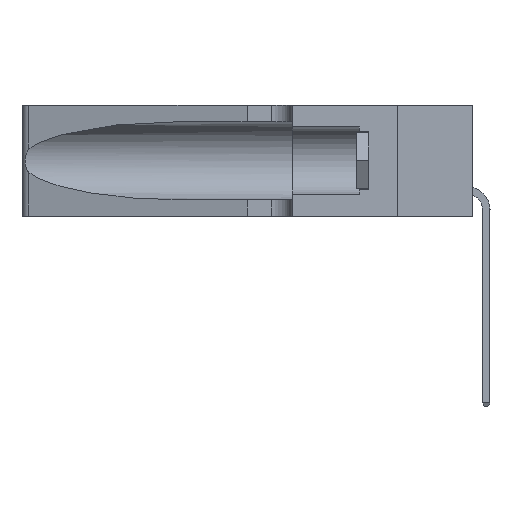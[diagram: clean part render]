
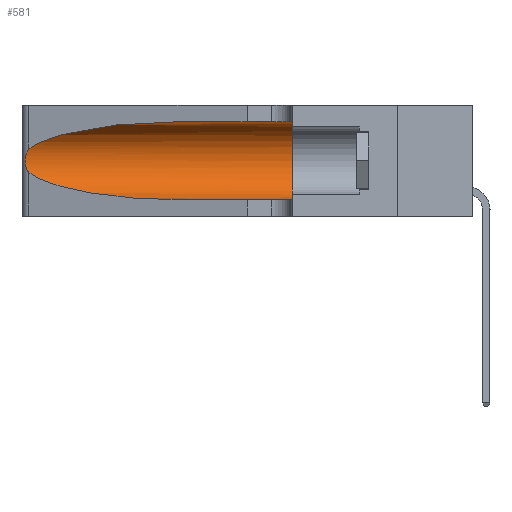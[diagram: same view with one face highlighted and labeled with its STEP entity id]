
A CAD part, left-side view. The second image highlights one B-rep face of the part: STEP entity #581.
In plain terms, the highlighted cylindrical face has radius 3.308 mm (diameter 6.617 mm), a partial arc.
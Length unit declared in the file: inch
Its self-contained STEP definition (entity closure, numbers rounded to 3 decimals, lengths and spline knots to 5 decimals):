
#228 = EDGE_CURVE ( 'NONE', #7086, #34649, #12203, .T. ) ;
#581 = ADVANCED_FACE ( 'NONE', ( #31337 ), #18608, .F. ) ;
#1753 = CARTESIAN_POINT ( 'NONE',  ( 0.25639, 1.23186, 0.15144 ) ) ;
#2280 =( BOUNDED_CURVE ( )  B_SPLINE_CURVE ( 3, ( #18532, #28367, #24804, #37638 ),
 .UNSPECIFIED., .F., .T. ) 
 B_SPLINE_CURVE_WITH_KNOTS ( ( 4, 4 ),
 ( 1.5708, 2.84003 ),
 .UNSPECIFIED. ) 
 CURVE ( )  GEOMETRIC_REPRESENTATION_ITEM ( )  RATIONAL_B_SPLINE_CURVE ( ( 1., 0.87, 0.87, 1. ) ) 
 REPRESENTATION_ITEM ( '' )  );
#4616 =( BOUNDED_CURVE ( )  B_SPLINE_CURVE ( 3, ( #35679, #6093, #32330, #28682 ),
 .UNSPECIFIED., .F., .F. ) 
 B_SPLINE_CURVE_WITH_KNOTS ( ( 4, 4 ),
 ( 3.44316, 4.71239 ),
 .UNSPECIFIED. ) 
 CURVE ( )  GEOMETRIC_REPRESENTATION_ITEM ( )  RATIONAL_B_SPLINE_CURVE ( ( 1., 0.87, 0.87, 1. ) ) 
 REPRESENTATION_ITEM ( '' )  );
#4776 = EDGE_CURVE ( 'NONE', #40085, #14666, #27175, .T. ) ;
#5029 = CARTESIAN_POINT ( 'NONE',  ( 0.25789, 1.23486, 0.15765 ) ) ;
#6093 = CARTESIAN_POINT ( 'NONE',  ( 0.2373, 1.15595, 0.08982 ) ) ;
#7025 = CARTESIAN_POINT ( 'NONE',  ( 0.25555, 1.22994, 0.2215 ) ) ;
#7086 = VERTEX_POINT ( 'NONE', #40949 ) ;
#7483 = ORIENTED_EDGE ( 'NONE', *, *, #8752, .T. ) ;
#8303 = CARTESIAN_POINT ( 'NONE',  ( 0.25555, 1.22993, 0.14849 ) ) ;
#8752 = EDGE_CURVE ( 'NONE', #40085, #7086, #2280, .T. ) ;
#9869 = CARTESIAN_POINT ( 'NONE',  ( 0.1305, 1.61858, 0.31525 ) ) ;
#10155 = ORIENTED_EDGE ( 'NONE', *, *, #11178, .T. ) ;
#11040 = VECTOR ( 'NONE', #30223, 39.37008 ) ;
#11178 = EDGE_CURVE ( 'NONE', #22840, #31168, #31362, .T. ) ;
#12203 = B_SPLINE_CURVE_WITH_KNOTS ( 'NONE', 3,
 ( #30043, #7025, #39729, #36611, #32995, #21078, #37460, #14257, #30453, #37320, #5029, #1753, #8303, #31007 ),
 .UNSPECIFIED., .F., .F.,
 ( 4, 2, 2, 2, 2, 2, 4 ),
 ( 0., 0.00027, 0.00053, 0.00107, 0.0016, 0.00187, 0.00214 ),
 .UNSPECIFIED. ) ;
#14257 = CARTESIAN_POINT ( 'NONE',  ( 0.26075, 1.23896, 0.178 ) ) ;
#14320 = CIRCLE ( 'NONE', #38857, 0.13025 ) ;
#14666 = VERTEX_POINT ( 'NONE', #34007 ) ;
#17607 = CARTESIAN_POINT ( 'NONE',  ( 0.25487, 1.22718, 0.14631 ) ) ;
#18046 = CARTESIAN_POINT ( 'NONE',  ( 0.1305, 1.61858, 0.185 ) ) ;
#18532 = CARTESIAN_POINT ( 'NONE',  ( 0.1305, 0.72297, 0.31525 ) ) ;
#18549 = VECTOR ( 'NONE', #25779, 39.37008 ) ;
#18608 = CYLINDRICAL_SURFACE ( 'NONE', #26297, 0.13025 ) ;
#18941 = CARTESIAN_POINT ( 'NONE',  ( 0.1305, 0.35, 0.185 ) ) ;
#19508 = DIRECTION ( 'NONE',  ( 0., 0., 1. ) ) ;
#20144 = CARTESIAN_POINT ( 'NONE',  ( 0.1305, 1.61858, 0.05475 ) ) ;
#21078 = CARTESIAN_POINT ( 'NONE',  ( 0.26018, 1.23835, 0.19895 ) ) ;
#22840 = VERTEX_POINT ( 'NONE', #32317 ) ;
#23544 = CARTESIAN_POINT ( 'NONE',  ( 0.1305, 0.35, 0.05475 ) ) ;
#23941 = EDGE_LOOP ( 'NONE', ( #7483, #37481, #27740, #10155, #29440, #30219 ) ) ;
#24804 = CARTESIAN_POINT ( 'NONE',  ( 0.2373, 1.15595, 0.28018 ) ) ;
#25779 = DIRECTION ( 'NONE',  ( 0., -1., 0. ) ) ;
#25839 = EDGE_CURVE ( 'NONE', #14666, #31168, #14320, .T. ) ;
#26297 = AXIS2_PLACEMENT_3D ( 'NONE', #18046, #27987, #31938 ) ;
#27175 = LINE ( 'NONE', #9869, #18549 ) ;
#27740 = ORIENTED_EDGE ( 'NONE', *, *, #39529, .T. ) ;
#27987 = DIRECTION ( 'NONE',  ( 0., -1., 0. ) ) ;
#28367 = CARTESIAN_POINT ( 'NONE',  ( 0.18966, 0.96281, 0.31525 ) ) ;
#28682 = CARTESIAN_POINT ( 'NONE',  ( 0.1305, 0.72297, 0.05475 ) ) ;
#29440 = ORIENTED_EDGE ( 'NONE', *, *, #25839, .F. ) ;
#30043 = CARTESIAN_POINT ( 'NONE',  ( 0.25487, 1.22718, 0.22369 ) ) ;
#30219 = ORIENTED_EDGE ( 'NONE', *, *, #4776, .F. ) ;
#30223 = DIRECTION ( 'NONE',  ( 0., -1., 0. ) ) ;
#30453 = CARTESIAN_POINT ( 'NONE',  ( 0.26017, 1.23833, 0.17102 ) ) ;
#31007 = CARTESIAN_POINT ( 'NONE',  ( 0.25487, 1.22718, 0.14631 ) ) ;
#31168 = VERTEX_POINT ( 'NONE', #23544 ) ;
#31337 = FACE_OUTER_BOUND ( 'NONE', #23941, .T. ) ;
#31362 = LINE ( 'NONE', #20144, #11040 ) ;
#31588 = CARTESIAN_POINT ( 'NONE',  ( 0.1305, 0.72297, 0.31525 ) ) ;
#31938 = DIRECTION ( 'NONE',  ( 0., 0., -1. ) ) ;
#32144 = DIRECTION ( 'NONE',  ( 0., 1., 0. ) ) ;
#32317 = CARTESIAN_POINT ( 'NONE',  ( 0.1305, 0.72297, 0.05475 ) ) ;
#32330 = CARTESIAN_POINT ( 'NONE',  ( 0.18966, 0.96281, 0.05475 ) ) ;
#32995 = CARTESIAN_POINT ( 'NONE',  ( 0.25854, 1.2359, 0.20912 ) ) ;
#34007 = CARTESIAN_POINT ( 'NONE',  ( 0.1305, 0.35, 0.31525 ) ) ;
#34649 = VERTEX_POINT ( 'NONE', #17607 ) ;
#35679 = CARTESIAN_POINT ( 'NONE',  ( 0.25487, 1.22718, 0.14631 ) ) ;
#36611 = CARTESIAN_POINT ( 'NONE',  ( 0.25787, 1.23484, 0.2124 ) ) ;
#37320 = CARTESIAN_POINT ( 'NONE',  ( 0.25856, 1.23593, 0.16098 ) ) ;
#37460 = CARTESIAN_POINT ( 'NONE',  ( 0.26075, 1.23896, 0.19203 ) ) ;
#37481 = ORIENTED_EDGE ( 'NONE', *, *, #228, .T. ) ;
#37638 = CARTESIAN_POINT ( 'NONE',  ( 0.25487, 1.22718, 0.22369 ) ) ;
#38857 = AXIS2_PLACEMENT_3D ( 'NONE', #18941, #32144, #19508 ) ;
#39529 = EDGE_CURVE ( 'NONE', #34649, #22840, #4616, .T. ) ;
#39729 = CARTESIAN_POINT ( 'NONE',  ( 0.25639, 1.23184, 0.21858 ) ) ;
#40085 = VERTEX_POINT ( 'NONE', #31588 ) ;
#40949 = CARTESIAN_POINT ( 'NONE',  ( 0.25487, 1.22718, 0.22369 ) ) ;
